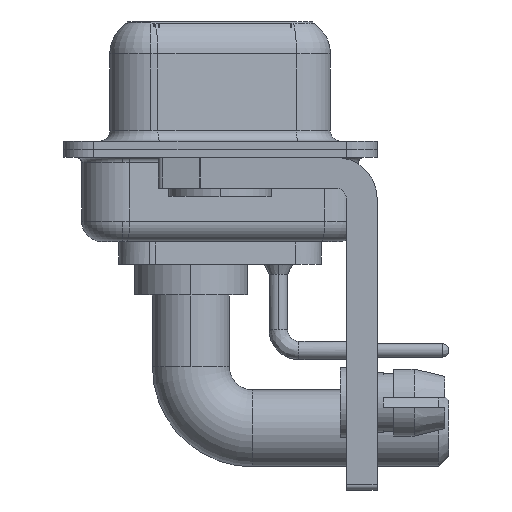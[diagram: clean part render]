
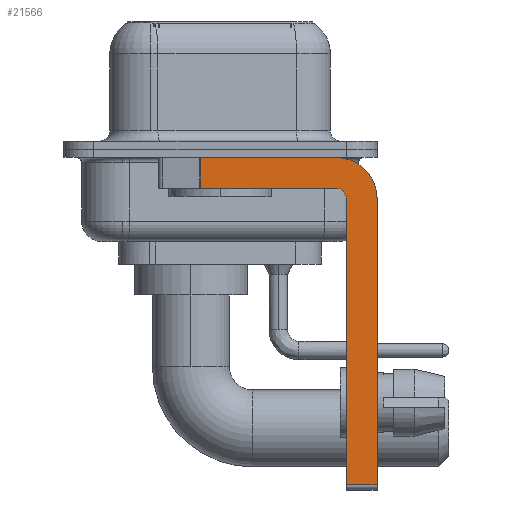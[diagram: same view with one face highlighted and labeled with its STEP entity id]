
A CAD part, left-side view. The second image highlights one B-rep face of the part: STEP entity #21566.
In plain terms, the highlighted planar face has unit normal (-1, 0, 0).
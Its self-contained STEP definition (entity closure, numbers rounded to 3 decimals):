
#6 = ORIENTED_EDGE ( 'NONE', *, *, #11428, .F. ) ;
#163 = CARTESIAN_POINT ( 'NONE',  ( -2.9, -5.65, -2.4 ) ) ;
#278 = PLANE ( 'NONE',  #9488 ) ;
#907 = ORIENTED_EDGE ( 'NONE', *, *, #18399, .T. ) ;
#1228 = CARTESIAN_POINT ( 'NONE',  ( -2.9, 0.978, -0.4 ) ) ;
#1240 = CARTESIAN_POINT ( 'NONE',  ( -2.9, 0.978, -1.9 ) ) ;
#1615 = ORIENTED_EDGE ( 'NONE', *, *, #6942, .F. ) ;
#2422 = CARTESIAN_POINT ( 'NONE',  ( -2.9, -6.15, -16.35 ) ) ;
#2725 = EDGE_LOOP ( 'NONE', ( #1615, #907, #6328, #15508, #21810, #7746, #6, #19417 ) ) ;
#2766 = AXIS2_PLACEMENT_3D ( 'NONE', #14970, #20352, #18356 ) ;
#3103 = DIRECTION ( 'NONE',  ( 0., 0., -1. ) ) ;
#3218 = LINE ( 'NONE', #13872, #17883 ) ;
#3904 = VERTEX_POINT ( 'NONE', #13462 ) ;
#4008 = LINE ( 'NONE', #7453, #5788 ) ;
#4913 = DIRECTION ( 'NONE',  ( 1., 0., 0. ) ) ;
#5139 = VECTOR ( 'NONE', #18860, 1000. ) ;
#5788 = VECTOR ( 'NONE', #13218, 1000. ) ;
#6328 = ORIENTED_EDGE ( 'NONE', *, *, #14616, .F. ) ;
#6441 = DIRECTION ( 'NONE',  ( 0., -1., 0. ) ) ;
#6629 = CARTESIAN_POINT ( 'NONE',  ( -2.9, -6.15, -2.4 ) ) ;
#6863 = VERTEX_POINT ( 'NONE', #19694 ) ;
#6942 = EDGE_CURVE ( 'NONE', #15376, #20458, #4008, .T. ) ;
#7239 = DIRECTION ( 'NONE',  ( 0., 0., 1. ) ) ;
#7453 = CARTESIAN_POINT ( 'NONE',  ( -2.9, 3., -0.4 ) ) ;
#7746 = ORIENTED_EDGE ( 'NONE', *, *, #18926, .T. ) ;
#8166 = LINE ( 'NONE', #11542, #5139 ) ;
#8501 = DIRECTION ( 'NONE',  ( 0., 0., -1. ) ) ;
#9204 = CARTESIAN_POINT ( 'NONE',  ( -2.9, -5.65, -1.9 ) ) ;
#9223 = DIRECTION ( 'NONE',  ( 1., 0., 0. ) ) ;
#9488 = AXIS2_PLACEMENT_3D ( 'NONE', #163, #9223, #22253 ) ;
#11382 = CARTESIAN_POINT ( 'NONE',  ( -2.9, -6.15, -16.6 ) ) ;
#11428 = EDGE_CURVE ( 'NONE', #6863, #3904, #19998, .T. ) ;
#11542 = CARTESIAN_POINT ( 'NONE',  ( -2.9, -5.65, -1.9 ) ) ;
#11716 = EDGE_CURVE ( 'NONE', #20458, #6863, #15298, .T. ) ;
#12114 = LINE ( 'NONE', #1240, #15172 ) ;
#12331 = CIRCLE ( 'NONE', #2766, 0.5 ) ;
#12822 = EDGE_CURVE ( 'NONE', #14374, #16724, #12331, .T. ) ;
#12926 = VECTOR ( 'NONE', #7239, 1000. ) ;
#13033 = CARTESIAN_POINT ( 'NONE',  ( -2.9, -5.65, -0.4 ) ) ;
#13218 = DIRECTION ( 'NONE',  ( 0., -1., 0. ) ) ;
#13346 = VERTEX_POINT ( 'NONE', #21006 ) ;
#13462 = CARTESIAN_POINT ( 'NONE',  ( -2.9, -7.65, -16.35 ) ) ;
#13872 = CARTESIAN_POINT ( 'NONE',  ( -2.9, -5.65, -16.35 ) ) ;
#14153 = CARTESIAN_POINT ( 'NONE',  ( -2.9, -7.65, -2.4 ) ) ;
#14374 = VERTEX_POINT ( 'NONE', #6629 ) ;
#14616 = EDGE_CURVE ( 'NONE', #16724, #13346, #8166, .T. ) ;
#14970 = CARTESIAN_POINT ( 'NONE',  ( -2.9, -5.65, -2.4 ) ) ;
#15172 = VECTOR ( 'NONE', #8501, 1000. ) ;
#15298 = CIRCLE ( 'NONE', #20634, 2. ) ;
#15376 = VERTEX_POINT ( 'NONE', #1228 ) ;
#15508 = ORIENTED_EDGE ( 'NONE', *, *, #12822, .F. ) ;
#16375 = LINE ( 'NONE', #11382, #12926 ) ;
#16724 = VERTEX_POINT ( 'NONE', #9204 ) ;
#17097 = VERTEX_POINT ( 'NONE', #2422 ) ;
#17883 = VECTOR ( 'NONE', #6441, 1000. ) ;
#18356 = DIRECTION ( 'NONE',  ( 0., 0., 1. ) ) ;
#18399 = EDGE_CURVE ( 'NONE', #15376, #13346, #12114, .T. ) ;
#18860 = DIRECTION ( 'NONE',  ( 0., 1., 0. ) ) ;
#18926 = EDGE_CURVE ( 'NONE', #17097, #3904, #3218, .T. ) ;
#19417 = ORIENTED_EDGE ( 'NONE', *, *, #11716, .F. ) ;
#19694 = CARTESIAN_POINT ( 'NONE',  ( -2.9, -7.65, -2.4 ) ) ;
#19736 = CARTESIAN_POINT ( 'NONE',  ( -2.9, -5.65, -2.4 ) ) ;
#19998 = LINE ( 'NONE', #14153, #22661 ) ;
#20352 = DIRECTION ( 'NONE',  ( -1., 0., 0. ) ) ;
#20458 = VERTEX_POINT ( 'NONE', #13033 ) ;
#20468 = FACE_OUTER_BOUND ( 'NONE', #2725, .T. ) ;
#20634 = AXIS2_PLACEMENT_3D ( 'NONE', #19736, #4913, #3103 ) ;
#20878 = EDGE_CURVE ( 'NONE', #17097, #14374, #16375, .T. ) ;
#21006 = CARTESIAN_POINT ( 'NONE',  ( -2.9, 0.978, -1.9 ) ) ;
#21566 = ADVANCED_FACE ( 'NONE', ( #20468 ), #278, .F. ) ;
#21810 = ORIENTED_EDGE ( 'NONE', *, *, #20878, .F. ) ;
#22253 = DIRECTION ( 'NONE',  ( 0., 0., -1. ) ) ;
#22661 = VECTOR ( 'NONE', #23333, 1000. ) ;
#23333 = DIRECTION ( 'NONE',  ( 0., 0., -1. ) ) ;
